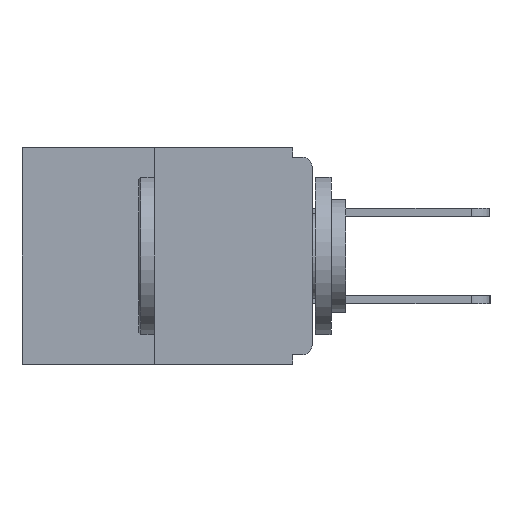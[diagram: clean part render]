
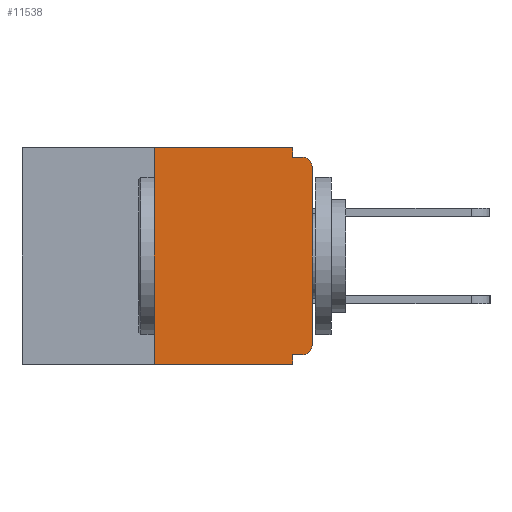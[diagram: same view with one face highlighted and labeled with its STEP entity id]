
A CAD part, left-side view. The second image highlights one B-rep face of the part: STEP entity #11538.
In plain terms, the highlighted planar face has unit normal (-1, 0, 0).
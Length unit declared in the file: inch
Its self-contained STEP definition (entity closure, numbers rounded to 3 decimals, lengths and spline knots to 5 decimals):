
#3 = EDGE_CURVE ( 'NONE', #7235, #19273, #16805, .T. ) ;
#387 = CARTESIAN_POINT ( 'NONE',  ( 0., 0.25, 0. ) ) ;
#1259 = ORIENTED_EDGE ( 'NONE', *, *, #3, .F. ) ;
#1309 = DIRECTION ( 'NONE',  ( 0., 0., -1. ) ) ;
#1799 = DIRECTION ( 'NONE',  ( 0., 1., 0. ) ) ;
#2236 = EDGE_CURVE ( 'NONE', #9753, #3498, #5536, .T. ) ;
#2504 = EDGE_CURVE ( 'NONE', #19273, #2790, #15923, .T. ) ;
#2577 = VECTOR ( 'NONE', #7587, 39.37008 ) ;
#2699 = LINE ( 'NONE', #13832, #18362 ) ;
#2790 = VERTEX_POINT ( 'NONE', #8182 ) ;
#2848 = LINE ( 'NONE', #387, #2577 ) ;
#3108 = VECTOR ( 'NONE', #10153, 39.37008 ) ;
#3315 = VECTOR ( 'NONE', #4556, 39.37008 ) ;
#3421 = CARTESIAN_POINT ( 'NONE',  ( 0., 0.46, 0. ) ) ;
#3498 = VERTEX_POINT ( 'NONE', #12456 ) ;
#4225 = DIRECTION ( 'NONE',  ( 1., 0., 0. ) ) ;
#4368 = PLANE ( 'NONE',  #21579 ) ;
#4556 = DIRECTION ( 'NONE',  ( 0., 0., -1. ) ) ;
#5195 = DIRECTION ( 'NONE',  ( 0., -1., 0. ) ) ;
#5323 = AXIS2_PLACEMENT_3D ( 'NONE', #14750, #13010, #14894 ) ;
#5469 = CARTESIAN_POINT ( 'NONE',  ( 0., 0., -0.313 ) ) ;
#5536 = LINE ( 'NONE', #10020, #21154 ) ;
#5696 = CIRCLE ( 'NONE', #5323, 0.015 ) ;
#5724 = CARTESIAN_POINT ( 'NONE',  ( 0., 0.031, -0.343 ) ) ;
#5855 = LINE ( 'NONE', #3421, #8691 ) ;
#6741 = AXIS2_PLACEMENT_3D ( 'NONE', #14591, #11339, #1309 ) ;
#6887 = FACE_OUTER_BOUND ( 'NONE', #18204, .T. ) ;
#7002 = VERTEX_POINT ( 'NONE', #10294 ) ;
#7235 = VERTEX_POINT ( 'NONE', #18250 ) ;
#7349 = VECTOR ( 'NONE', #7615, 39.37008 ) ;
#7507 = ORIENTED_EDGE ( 'NONE', *, *, #14850, .T. ) ;
#7587 = DIRECTION ( 'NONE',  ( 0., 0., 1. ) ) ;
#7615 = DIRECTION ( 'NONE',  ( 0., 0., -1. ) ) ;
#8182 = CARTESIAN_POINT ( 'NONE',  ( 0., 0.031, -0.343 ) ) ;
#8256 = VERTEX_POINT ( 'NONE', #9237 ) ;
#8691 = VECTOR ( 'NONE', #5195, 39.37008 ) ;
#8880 = CARTESIAN_POINT ( 'NONE',  ( 0., 0.015, -0.015 ) ) ;
#9237 = CARTESIAN_POINT ( 'NONE',  ( 0., 0.25, -0.343 ) ) ;
#9464 = EDGE_CURVE ( 'NONE', #7002, #10747, #12717, .T. ) ;
#9753 = VERTEX_POINT ( 'NONE', #5469 ) ;
#9937 = ORIENTED_EDGE ( 'NONE', *, *, #9464, .F. ) ;
#10020 = CARTESIAN_POINT ( 'NONE',  ( 0., 0., 0. ) ) ;
#10153 = DIRECTION ( 'NONE',  ( 0., -1., 0. ) ) ;
#10294 = CARTESIAN_POINT ( 'NONE',  ( 0., 0.031, 0. ) ) ;
#10747 = VERTEX_POINT ( 'NONE', #11707 ) ;
#11339 = DIRECTION ( 'NONE',  ( -1., 0., 0. ) ) ;
#11538 = ADVANCED_FACE ( 'NONE', ( #6887 ), #4368, .F. ) ;
#11707 = CARTESIAN_POINT ( 'NONE',  ( 0., 0.031, -0.015 ) ) ;
#12035 = CARTESIAN_POINT ( 'NONE',  ( 0., 0.46, -0.343 ) ) ;
#12387 = VECTOR ( 'NONE', #1799, 39.37008 ) ;
#12456 = CARTESIAN_POINT ( 'NONE',  ( 0., 0., -0.03 ) ) ;
#12520 = CARTESIAN_POINT ( 'NONE',  ( 0., 0.25, 0. ) ) ;
#12717 = LINE ( 'NONE', #18479, #3315 ) ;
#12845 = ORIENTED_EDGE ( 'NONE', *, *, #16221, .F. ) ;
#12903 = DIRECTION ( 'NONE',  ( 0., 0., -1. ) ) ;
#13010 = DIRECTION ( 'NONE',  ( -1., 0., 0. ) ) ;
#13568 = EDGE_CURVE ( 'NONE', #8256, #2790, #15874, .T. ) ;
#13647 = VERTEX_POINT ( 'NONE', #8880 ) ;
#13699 = EDGE_CURVE ( 'NONE', #8256, #20130, #2848, .T. ) ;
#13832 = CARTESIAN_POINT ( 'NONE',  ( 0., 0., -0.015 ) ) ;
#14006 = CIRCLE ( 'NONE', #6741, 0.015 ) ;
#14062 = DIRECTION ( 'NONE',  ( 0., -1., 0. ) ) ;
#14193 = CARTESIAN_POINT ( 'NONE',  ( 0., 0.46, 0. ) ) ;
#14591 = CARTESIAN_POINT ( 'NONE',  ( 0., 0.015, -0.03 ) ) ;
#14750 = CARTESIAN_POINT ( 'NONE',  ( 0., 0.015, -0.313 ) ) ;
#14850 = EDGE_CURVE ( 'NONE', #7235, #9753, #5696, .T. ) ;
#14866 = EDGE_CURVE ( 'NONE', #3498, #13647, #14006, .T. ) ;
#14894 = DIRECTION ( 'NONE',  ( 0., 0., -1. ) ) ;
#15001 = CARTESIAN_POINT ( 'NONE',  ( 0., 0., -0.328 ) ) ;
#15582 = ORIENTED_EDGE ( 'NONE', *, *, #14866, .T. ) ;
#15874 = LINE ( 'NONE', #12035, #3108 ) ;
#15923 = LINE ( 'NONE', #5724, #7349 ) ;
#16221 = EDGE_CURVE ( 'NONE', #10747, #13647, #2699, .T. ) ;
#16284 = ORIENTED_EDGE ( 'NONE', *, *, #2236, .T. ) ;
#16805 = LINE ( 'NONE', #15001, #12387 ) ;
#17691 = ORIENTED_EDGE ( 'NONE', *, *, #13568, .T. ) ;
#17706 = EDGE_CURVE ( 'NONE', #20130, #7002, #5855, .T. ) ;
#17837 = ORIENTED_EDGE ( 'NONE', *, *, #17706, .F. ) ;
#18204 = EDGE_LOOP ( 'NONE', ( #17837, #20155, #17691, #20422, #1259, #7507, #16284, #15582, #12845, #9937 ) ) ;
#18223 = DIRECTION ( 'NONE',  ( 0., 0., 1. ) ) ;
#18250 = CARTESIAN_POINT ( 'NONE',  ( 0., 0.015, -0.328 ) ) ;
#18362 = VECTOR ( 'NONE', #14062, 39.37008 ) ;
#18479 = CARTESIAN_POINT ( 'NONE',  ( 0., 0.031, 0. ) ) ;
#19056 = CARTESIAN_POINT ( 'NONE',  ( 0., 0.031, -0.328 ) ) ;
#19273 = VERTEX_POINT ( 'NONE', #19056 ) ;
#20130 = VERTEX_POINT ( 'NONE', #12520 ) ;
#20155 = ORIENTED_EDGE ( 'NONE', *, *, #13699, .F. ) ;
#20422 = ORIENTED_EDGE ( 'NONE', *, *, #2504, .F. ) ;
#21154 = VECTOR ( 'NONE', #18223, 39.37008 ) ;
#21579 = AXIS2_PLACEMENT_3D ( 'NONE', #14193, #4225, #12903 ) ;
